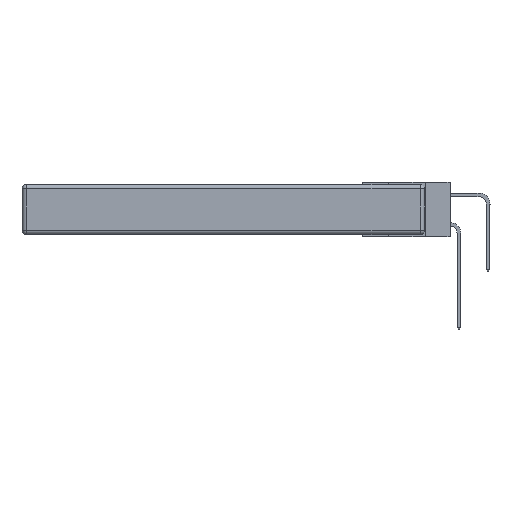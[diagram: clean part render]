
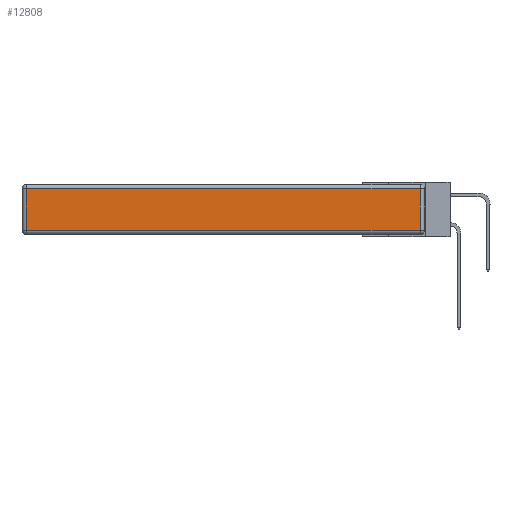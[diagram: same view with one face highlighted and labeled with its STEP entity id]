
A CAD part, left-side view. The second image highlights one B-rep face of the part: STEP entity #12808.
In plain terms, the highlighted planar face has unit normal (-1, 0, 0).
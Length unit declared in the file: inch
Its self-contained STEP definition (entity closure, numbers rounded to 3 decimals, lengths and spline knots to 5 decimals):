
#97 = DIRECTION ( 'NONE',  ( 0., 0., -1. ) ) ;
#418 = EDGE_CURVE ( 'NONE', #7809, #9409, #13278, .T. ) ;
#530 = ORIENTED_EDGE ( 'NONE', *, *, #13268, .T. ) ;
#1289 = ORIENTED_EDGE ( 'NONE', *, *, #11223, .T. ) ;
#1652 = VERTEX_POINT ( 'NONE', #4046 ) ;
#1752 = CARTESIAN_POINT ( 'NONE',  ( 0., 0.03, -0.343 ) ) ;
#2196 = DIRECTION ( 'NONE',  ( 0., 0., 1. ) ) ;
#2977 = DIRECTION ( 'NONE',  ( 0., 1., 0. ) ) ;
#3595 = VECTOR ( 'NONE', #8991, 39.37008 ) ;
#4046 = CARTESIAN_POINT ( 'NONE',  ( 0., 0.03, -0.03 ) ) ;
#4206 = PLANE ( 'NONE',  #7737 ) ;
#4323 = ORIENTED_EDGE ( 'NONE', *, *, #418, .T. ) ;
#5588 = EDGE_LOOP ( 'NONE', ( #4323, #530, #6895, #1289 ) ) ;
#5863 = LINE ( 'NONE', #1752, #11301 ) ;
#6010 = VERTEX_POINT ( 'NONE', #12494 ) ;
#6246 = DIRECTION ( 'NONE',  ( 0., 0., 1. ) ) ;
#6494 = CARTESIAN_POINT ( 'NONE',  ( 0., 0.03, -0.313 ) ) ;
#6895 = ORIENTED_EDGE ( 'NONE', *, *, #8545, .T. ) ;
#7092 = FACE_OUTER_BOUND ( 'NONE', #5588, .T. ) ;
#7479 = LINE ( 'NONE', #8882, #13520 ) ;
#7737 = AXIS2_PLACEMENT_3D ( 'NONE', #13061, #9736, #2196 ) ;
#7809 = VERTEX_POINT ( 'NONE', #12847 ) ;
#8545 = EDGE_CURVE ( 'NONE', #1652, #6010, #13596, .T. ) ;
#8731 = VECTOR ( 'NONE', #2977, 39.37008 ) ;
#8882 = CARTESIAN_POINT ( 'NONE',  ( 0., 2.72, -0.343 ) ) ;
#8991 = DIRECTION ( 'NONE',  ( 0., -1., 0. ) ) ;
#9409 = VERTEX_POINT ( 'NONE', #6494 ) ;
#9736 = DIRECTION ( 'NONE',  ( -1., 0., 0. ) ) ;
#11223 = EDGE_CURVE ( 'NONE', #6010, #7809, #7479, .T. ) ;
#11301 = VECTOR ( 'NONE', #6246, 39.37008 ) ;
#11844 = CARTESIAN_POINT ( 'NONE',  ( 0., 2.75, -0.03 ) ) ;
#12131 = CARTESIAN_POINT ( 'NONE',  ( 0., 0., -0.313 ) ) ;
#12494 = CARTESIAN_POINT ( 'NONE',  ( 0., 2.72, -0.03 ) ) ;
#12808 = ADVANCED_FACE ( 'NONE', ( #7092 ), #4206, .T. ) ;
#12847 = CARTESIAN_POINT ( 'NONE',  ( 0., 2.72, -0.313 ) ) ;
#13061 = CARTESIAN_POINT ( 'NONE',  ( 0., 0., -0.343 ) ) ;
#13268 = EDGE_CURVE ( 'NONE', #9409, #1652, #5863, .T. ) ;
#13278 = LINE ( 'NONE', #12131, #3595 ) ;
#13520 = VECTOR ( 'NONE', #97, 39.37008 ) ;
#13596 = LINE ( 'NONE', #11844, #8731 ) ;
